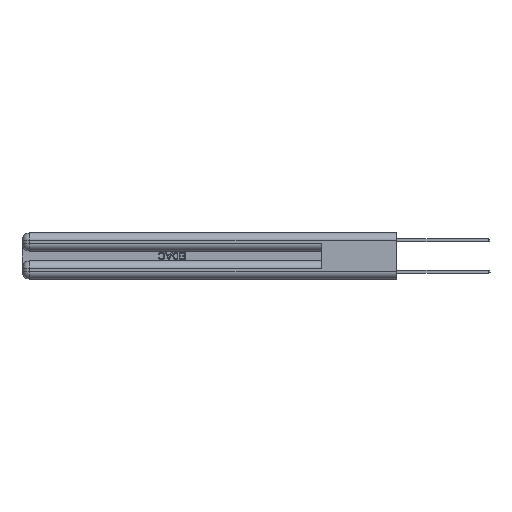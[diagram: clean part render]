
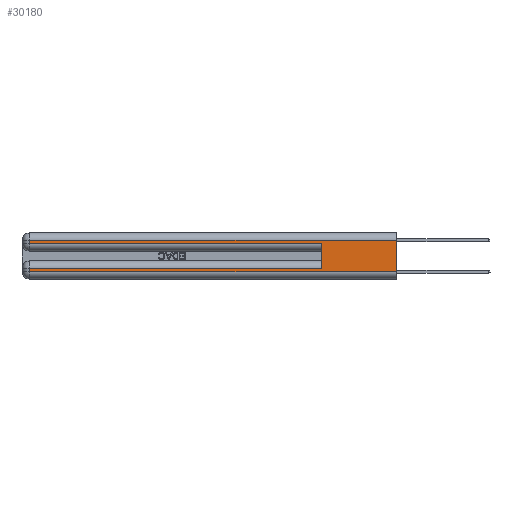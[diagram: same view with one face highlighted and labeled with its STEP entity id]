
A CAD part, left-side view. The second image highlights one B-rep face of the part: STEP entity #30180.
In plain terms, the highlighted planar face has unit normal (-1, 0, 0).
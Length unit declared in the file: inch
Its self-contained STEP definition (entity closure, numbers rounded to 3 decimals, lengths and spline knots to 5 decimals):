
#515 = DIRECTION ( 'NONE',  ( 0., 0., -1. ) ) ;
#966 = DIRECTION ( 'NONE',  ( 1., 0., 0. ) ) ;
#1310 = CARTESIAN_POINT ( 'NONE',  ( 0., 2.94, 0.285 ) ) ;
#1608 = CARTESIAN_POINT ( 'NONE',  ( 0., 0., 0.06 ) ) ;
#2252 = CARTESIAN_POINT ( 'NONE',  ( 0., 0.6, 0.085 ) ) ;
#2719 = VECTOR ( 'NONE', #515, 39.37008 ) ;
#3125 = LINE ( 'NONE', #25588, #29561 ) ;
#4584 = CARTESIAN_POINT ( 'NONE',  ( 0., 0.6, 0.285 ) ) ;
#5264 = EDGE_CURVE ( 'NONE', #20803, #13380, #10283, .T. ) ;
#5516 = EDGE_CURVE ( 'NONE', #26437, #19421, #3125, .T. ) ;
#6344 = CARTESIAN_POINT ( 'NONE',  ( 0., 0., 0.37 ) ) ;
#6466 = DIRECTION ( 'NONE',  ( 0., 1., 0. ) ) ;
#6555 = VECTOR ( 'NONE', #14324, 39.37008 ) ;
#6732 = CARTESIAN_POINT ( 'NONE',  ( 0., 2.94, 0.37 ) ) ;
#6980 = ORIENTED_EDGE ( 'NONE', *, *, #32196, .T. ) ;
#7325 = VERTEX_POINT ( 'NONE', #1310 ) ;
#8137 = VECTOR ( 'NONE', #17903, 39.37008 ) ;
#8453 = ORIENTED_EDGE ( 'NONE', *, *, #5264, .F. ) ;
#9286 = CARTESIAN_POINT ( 'NONE',  ( 0., 0., 0.085 ) ) ;
#9413 = DIRECTION ( 'NONE',  ( 0., 0., -1. ) ) ;
#10283 = LINE ( 'NONE', #19500, #2719 ) ;
#10480 = CARTESIAN_POINT ( 'NONE',  ( 0., 0., 0.31 ) ) ;
#13288 = DIRECTION ( 'NONE',  ( 0., -1., 0. ) ) ;
#13380 = VERTEX_POINT ( 'NONE', #1608 ) ;
#14085 = VERTEX_POINT ( 'NONE', #2252 ) ;
#14246 = DIRECTION ( 'NONE',  ( 0., 0., 1. ) ) ;
#14324 = DIRECTION ( 'NONE',  ( 0., 1., 0. ) ) ;
#14403 = VERTEX_POINT ( 'NONE', #24752 ) ;
#14480 = CARTESIAN_POINT ( 'NONE',  ( 0., 0.6, 0.145 ) ) ;
#15804 = LINE ( 'NONE', #22693, #6555 ) ;
#17521 = CARTESIAN_POINT ( 'NONE',  ( 0., 2.94, 0.085 ) ) ;
#17647 = EDGE_CURVE ( 'NONE', #7325, #28366, #18896, .T. ) ;
#17903 = DIRECTION ( 'NONE',  ( 0., 0., -1. ) ) ;
#18165 = ORIENTED_EDGE ( 'NONE', *, *, #5516, .T. ) ;
#18193 = ORIENTED_EDGE ( 'NONE', *, *, #33410, .T. ) ;
#18896 = LINE ( 'NONE', #29264, #31887 ) ;
#18998 = ORIENTED_EDGE ( 'NONE', *, *, #27668, .T. ) ;
#19421 = VERTEX_POINT ( 'NONE', #28621 ) ;
#19500 = CARTESIAN_POINT ( 'NONE',  ( 0., 0., 0.37 ) ) ;
#20342 = EDGE_LOOP ( 'NONE', ( #8453, #6980, #18998, #22729, #23138, #18193, #18165, #25216 ) ) ;
#20510 = VECTOR ( 'NONE', #13288, 39.37008 ) ;
#20803 = VERTEX_POINT ( 'NONE', #10480 ) ;
#22693 = CARTESIAN_POINT ( 'NONE',  ( 0., 0., 0.31 ) ) ;
#22729 = ORIENTED_EDGE ( 'NONE', *, *, #17647, .T. ) ;
#23138 = ORIENTED_EDGE ( 'NONE', *, *, #23757, .F. ) ;
#23757 = EDGE_CURVE ( 'NONE', #14085, #28366, #28071, .T. ) ;
#24065 = LINE ( 'NONE', #9286, #25362 ) ;
#24112 = DIRECTION ( 'NONE',  ( 0., -1., 0. ) ) ;
#24752 = CARTESIAN_POINT ( 'NONE',  ( 0., 2.94, 0.31 ) ) ;
#25216 = ORIENTED_EDGE ( 'NONE', *, *, #30412, .T. ) ;
#25362 = VECTOR ( 'NONE', #6466, 39.37008 ) ;
#25470 = PLANE ( 'NONE',  #32016 ) ;
#25588 = CARTESIAN_POINT ( 'NONE',  ( 0., 2.94, 0.37 ) ) ;
#26052 = DIRECTION ( 'NONE',  ( 0., 0., -1. ) ) ;
#26437 = VERTEX_POINT ( 'NONE', #17521 ) ;
#26600 = LINE ( 'NONE', #6732, #8137 ) ;
#27242 = LINE ( 'NONE', #31198, #20510 ) ;
#27668 = EDGE_CURVE ( 'NONE', #14403, #7325, #26600, .T. ) ;
#28071 = LINE ( 'NONE', #14480, #30193 ) ;
#28366 = VERTEX_POINT ( 'NONE', #4584 ) ;
#28621 = CARTESIAN_POINT ( 'NONE',  ( 0., 2.94, 0.06 ) ) ;
#29264 = CARTESIAN_POINT ( 'NONE',  ( 0., 0., 0.285 ) ) ;
#29561 = VECTOR ( 'NONE', #26052, 39.37008 ) ;
#30180 = ADVANCED_FACE ( 'NONE', ( #33953 ), #25470, .F. ) ;
#30193 = VECTOR ( 'NONE', #14246, 39.37008 ) ;
#30412 = EDGE_CURVE ( 'NONE', #19421, #13380, #27242, .T. ) ;
#31198 = CARTESIAN_POINT ( 'NONE',  ( 0., 0., 0.06 ) ) ;
#31887 = VECTOR ( 'NONE', #24112, 39.37008 ) ;
#32016 = AXIS2_PLACEMENT_3D ( 'NONE', #6344, #966, #9413 ) ;
#32196 = EDGE_CURVE ( 'NONE', #20803, #14403, #15804, .T. ) ;
#33410 = EDGE_CURVE ( 'NONE', #14085, #26437, #24065, .T. ) ;
#33953 = FACE_OUTER_BOUND ( 'NONE', #20342, .T. ) ;
